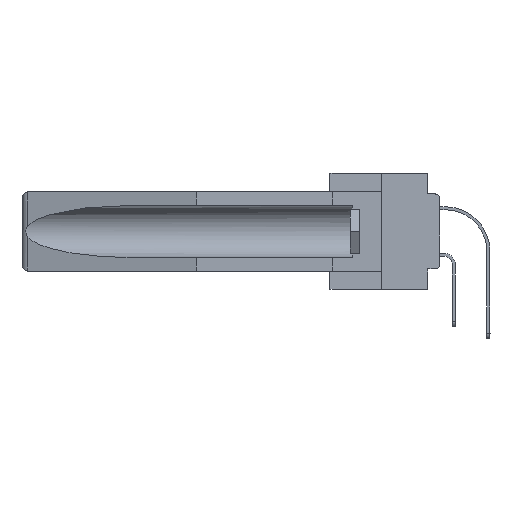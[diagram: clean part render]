
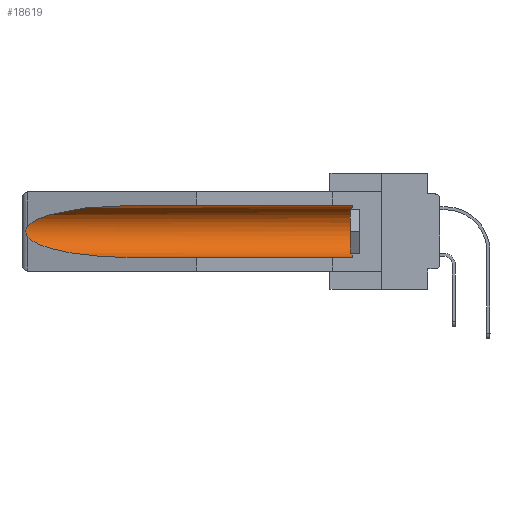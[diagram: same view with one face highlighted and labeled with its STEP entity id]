
A CAD part, left-side view. The second image highlights one B-rep face of the part: STEP entity #18619.
In plain terms, the highlighted cylindrical face has radius 2.857 mm (diameter 5.715 mm), a partial arc.
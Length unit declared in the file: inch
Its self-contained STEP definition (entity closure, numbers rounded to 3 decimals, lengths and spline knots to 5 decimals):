
#137 = DIRECTION ( 'NONE',  ( 0., 1., 0. ) ) ;
#212 = CARTESIAN_POINT ( 'NONE',  ( 0.155, 0.126, -0.284 ) ) ;
#1375 = CARTESIAN_POINT ( 'NONE',  ( 0.21114, 1.30732, -0.284 ) ) ;
#1803 = VERTEX_POINT ( 'NONE', #27267 ) ;
#1838 = VERTEX_POINT ( 'NONE', #30016 ) ;
#2434 = EDGE_CURVE ( 'NONE', #9849, #11415, #15627, .T. ) ;
#3832 = AXIS2_PLACEMENT_3D ( 'NONE', #29660, #18769, #18241 ) ;
#4080 = FACE_OUTER_BOUND ( 'NONE', #30784, .T. ) ;
#4127 = CARTESIAN_POINT ( 'NONE',  ( 0.26655, 1.53094, -0.18657 ) ) ;
#4362 = CARTESIAN_POINT ( 'NONE',  ( 0.155, -0.30754, -0.059 ) ) ;
#4543 = LINE ( 'NONE', #4362, #18330 ) ;
#5183 = EDGE_CURVE ( 'NONE', #1838, #24137, #4543, .T. ) ;
#6321 = ORIENTED_EDGE ( 'NONE', *, *, #30408, .F. ) ;
#9014 = CARTESIAN_POINT ( 'NONE',  ( 0.25451, 1.48313, -0.24835 ) ) ;
#9212 = CARTESIAN_POINT ( 'NONE',  ( 0.26537, 1.52718, -0.19328 ) ) ;
#9849 = VERTEX_POINT ( 'NONE', #14605 ) ;
#10166 = DIRECTION ( 'NONE',  ( 0., 1., 0. ) ) ;
#11211 = ORIENTED_EDGE ( 'NONE', *, *, #5183, .T. ) ;
#11414 = AXIS2_PLACEMENT_3D ( 'NONE', #18419, #18034, #12413 ) ;
#11415 = VERTEX_POINT ( 'NONE', #35892 ) ;
#12413 = DIRECTION ( 'NONE',  ( 0., 0., 1. ) ) ;
#12420 = ORIENTED_EDGE ( 'NONE', *, *, #21954, .T. ) ;
#13042 = CARTESIAN_POINT ( 'NONE',  ( 0.155, 1.07973, -0.059 ) ) ;
#13385 = ORIENTED_EDGE ( 'NONE', *, *, #2434, .T. ) ;
#13704 = CIRCLE ( 'NONE', #11414, 0.1125 ) ;
#14605 = CARTESIAN_POINT ( 'NONE',  ( 0.26537, 1.52718, -0.19328 ) ) ;
#14807 = VECTOR ( 'NONE', #137, 39.37008 ) ;
#14849 = CARTESIAN_POINT ( 'NONE',  ( 0.2673, 1.53269, -0.17917 ) ) ;
#15017 = CARTESIAN_POINT ( 'NONE',  ( 0.26597, 1.52961, -0.15275 ) ) ;
#15320 = VERTEX_POINT ( 'NONE', #212 ) ;
#15627 =( BOUNDED_CURVE ( )  B_SPLINE_CURVE ( 3, ( #28626, #9014, #1375, #23543 ),
 .UNSPECIFIED., .F., .F. ) 
 B_SPLINE_CURVE_WITH_KNOTS ( ( 4, 4 ),
 ( 0.1948, 1.5708 ),
 .UNSPECIFIED. ) 
 CURVE ( )  GEOMETRIC_REPRESENTATION_ITEM ( )  RATIONAL_B_SPLINE_CURVE ( ( 1., 0.848, 0.848, 1. ) ) 
 REPRESENTATION_ITEM ( '' )  );
#18034 = DIRECTION ( 'NONE',  ( 0., -1., 0. ) ) ;
#18241 = DIRECTION ( 'NONE',  ( 0., 0., 1. ) ) ;
#18330 = VECTOR ( 'NONE', #10166, 39.37008 ) ;
#18389 = CARTESIAN_POINT ( 'NONE',  ( 0.25451, 1.48313, -0.09465 ) ) ;
#18419 = CARTESIAN_POINT ( 'NONE',  ( 0.155, 0.126, -0.1715 ) ) ;
#18619 = ADVANCED_FACE ( 'NONE', ( #4080 ), #23516, .F. ) ;
#18769 = DIRECTION ( 'NONE',  ( 0., 1., 0. ) ) ;
#20473 = CARTESIAN_POINT ( 'NONE',  ( 0.26597, 1.5296, -0.19026 ) ) ;
#21954 = EDGE_CURVE ( 'NONE', #15320, #1838, #13704, .T. ) ;
#22311 = LINE ( 'NONE', #25221, #14807 ) ;
#23044 = CARTESIAN_POINT ( 'NONE',  ( 0.2673, 1.5327, -0.16383 ) ) ;
#23202 = CARTESIAN_POINT ( 'NONE',  ( 0.2675, 1.53308, -0.16763 ) ) ;
#23516 = CYLINDRICAL_SURFACE ( 'NONE', #3832, 0.1125 ) ;
#23543 = CARTESIAN_POINT ( 'NONE',  ( 0.155, 1.07973, -0.284 ) ) ;
#23575 = CARTESIAN_POINT ( 'NONE',  ( 0.26537, 1.52718, -0.14972 ) ) ;
#24137 = VERTEX_POINT ( 'NONE', #13042 ) ;
#24506 = ORIENTED_EDGE ( 'NONE', *, *, #30540, .T. ) ;
#24991 = EDGE_CURVE ( 'NONE', #24137, #1803, #28189, .T. ) ;
#25221 = CARTESIAN_POINT ( 'NONE',  ( 0.155, -0.30754, -0.284 ) ) ;
#25505 = ORIENTED_EDGE ( 'NONE', *, *, #24991, .T. ) ;
#27267 = CARTESIAN_POINT ( 'NONE',  ( 0.26537, 1.52718, -0.14972 ) ) ;
#28189 =( BOUNDED_CURVE ( )  B_SPLINE_CURVE ( 3, ( #32367, #35284, #18389, #35097 ),
 .UNSPECIFIED., .F., .F. ) 
 B_SPLINE_CURVE_WITH_KNOTS ( ( 4, 4 ),
 ( 4.71239, 6.08839 ),
 .UNSPECIFIED. ) 
 CURVE ( )  GEOMETRIC_REPRESENTATION_ITEM ( )  RATIONAL_B_SPLINE_CURVE ( ( 1., 0.848, 0.848, 1. ) ) 
 REPRESENTATION_ITEM ( '' )  );
#28626 = CARTESIAN_POINT ( 'NONE',  ( 0.26537, 1.52718, -0.19328 ) ) ;
#28662 = CARTESIAN_POINT ( 'NONE',  ( 0.26654, 1.53092, -0.15636 ) ) ;
#29019 = CARTESIAN_POINT ( 'NONE',  ( 0.2675, 1.53308, -0.17534 ) ) ;
#29660 = CARTESIAN_POINT ( 'NONE',  ( 0.155, -0.30754, -0.1715 ) ) ;
#30016 = CARTESIAN_POINT ( 'NONE',  ( 0.155, 0.126, -0.059 ) ) ;
#30408 = EDGE_CURVE ( 'NONE', #15320, #11415, #22311, .T. ) ;
#30540 = EDGE_CURVE ( 'NONE', #1803, #9849, #33619, .T. ) ;
#30784 = EDGE_LOOP ( 'NONE', ( #25505, #24506, #13385, #6321, #12420, #11211 ) ) ;
#32367 = CARTESIAN_POINT ( 'NONE',  ( 0.155, 1.07973, -0.059 ) ) ;
#33619 = B_SPLINE_CURVE_WITH_KNOTS ( 'NONE', 3,
 ( #23575, #15017, #28662, #23044, #23202, #29019, #14849, #4127, #20473, #9212 ),
 .UNSPECIFIED., .F., .F.,
 ( 4, 2, 2, 2, 4 ),
 ( 0., 0.00029, 0.00058, 0.00087, 0.00117 ),
 .UNSPECIFIED. ) ;
#35097 = CARTESIAN_POINT ( 'NONE',  ( 0.26537, 1.52718, -0.14972 ) ) ;
#35284 = CARTESIAN_POINT ( 'NONE',  ( 0.21114, 1.30732, -0.059 ) ) ;
#35892 = CARTESIAN_POINT ( 'NONE',  ( 0.155, 1.07973, -0.284 ) ) ;
